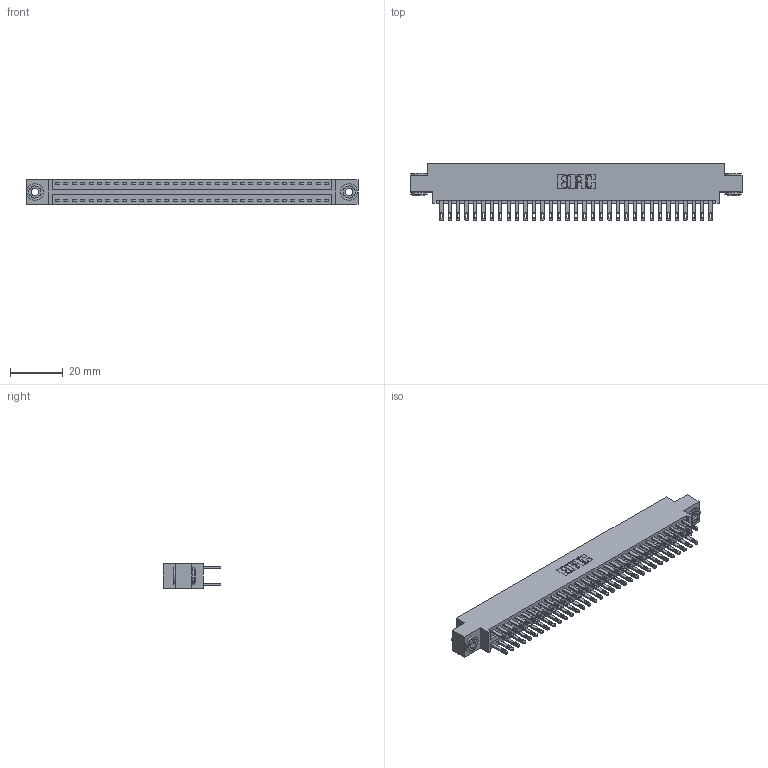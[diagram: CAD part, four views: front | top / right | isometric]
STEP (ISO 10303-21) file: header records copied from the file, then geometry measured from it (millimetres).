
FILE_DESCRIPTION (( 'STEP AP203' ), '1' );
FILE_NAME ('896-066-500-803.STEP', '2021-07-28T00:55:48', ( '' ), ( '' ), 'SwSTEP 2.0', 'SolidWorks 2020', '' );
FILE_SCHEMA (( 'CONFIG_CONTROL_DESIGN' ));
Length unit declared in the file: inch
Products named in the file (4): 846 Part_0.170 Offset - 0.156 Dia-TH; 345-250-002_345-250-002-102; 896-066-500-803; 345-292-001_345-293-100
Assembly tree (69 placements, depth 2):
  896-066-500-803
    846 Part_0.170 Offset - 0.156 Dia-TH
    345-292-001_345-293-100  x66
    345-250-002_345-250-002-102  x2
Bounding box: 125.35 x 21.84 x 9.4 mm (x, y, z)
Volume: 12219.6 mm3; surface area: 17739.9 mm2
Topology: 69 solids, 69 shells, 3332 faces, 10119 edges, 6742 vertices
Faces by surface type: plane 2004, cylinder 1320, cone 8
Entity records: 23460 total; most frequent: CARTESIAN_POINT 3855, ORIENTED_EDGE 3782, DIRECTION 3481, EDGE_CURVE 1891, LINE 1599, VECTOR 1599, VERTEX_POINT 1258, AXIS2_PLACEMENT_3D 941
